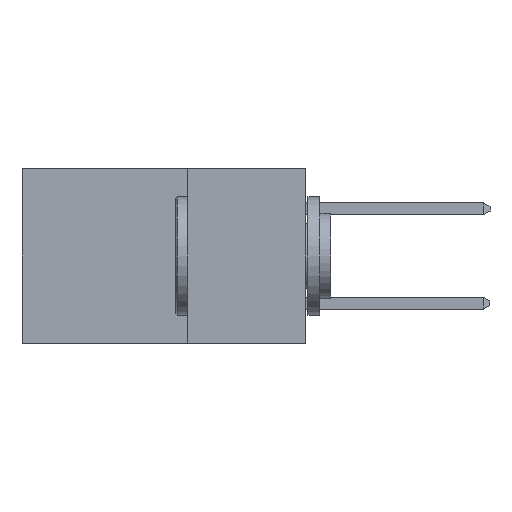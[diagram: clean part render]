
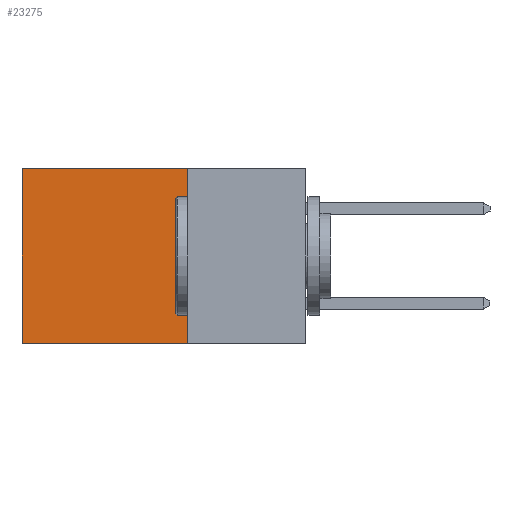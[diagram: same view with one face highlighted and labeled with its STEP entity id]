
A CAD part, left-side view. The second image highlights one B-rep face of the part: STEP entity #23275.
In plain terms, the highlighted planar face has unit normal (-1, 0, 0).
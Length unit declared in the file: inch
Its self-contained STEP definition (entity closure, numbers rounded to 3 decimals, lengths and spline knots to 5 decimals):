
#41 = ORIENTED_EDGE ( 'NONE', *, *, #3995, .F. ) ;
#1849 = CARTESIAN_POINT ( 'NONE',  ( 0.298, 0.25, 0. ) ) ;
#2735 = VERTEX_POINT ( 'NONE', #5864 ) ;
#3995 = EDGE_CURVE ( 'NONE', #4133, #2735, #20328, .T. ) ;
#4133 = VERTEX_POINT ( 'NONE', #1849 ) ;
#5017 = CARTESIAN_POINT ( 'NONE',  ( 0.298, 0.25, -0.37 ) ) ;
#5154 = ORIENTED_EDGE ( 'NONE', *, *, #13504, .T. ) ;
#5864 = CARTESIAN_POINT ( 'NONE',  ( 0.298, 0.25, -0.37 ) ) ;
#6428 = DIRECTION ( 'NONE',  ( 0., 1., 0. ) ) ;
#7084 = VECTOR ( 'NONE', #25562, 39.37008 ) ;
#7265 = DIRECTION ( 'NONE',  ( 0., 1., 0. ) ) ;
#7666 = VERTEX_POINT ( 'NONE', #19986 ) ;
#8743 = VECTOR ( 'NONE', #25901, 39.37008 ) ;
#9275 = ORIENTED_EDGE ( 'NONE', *, *, #20867, .F. ) ;
#10315 = VECTOR ( 'NONE', #6428, 39.37008 ) ;
#11048 = DIRECTION ( 'NONE',  ( 0., 0., -1. ) ) ;
#13504 = EDGE_CURVE ( 'NONE', #4133, #24951, #21853, .T. ) ;
#14989 = PLANE ( 'NONE',  #20465 ) ;
#16361 = CARTESIAN_POINT ( 'NONE',  ( 0.298, 0.6, 0. ) ) ;
#16399 = VECTOR ( 'NONE', #7265, 39.37008 ) ;
#16964 = CARTESIAN_POINT ( 'NONE',  ( 0.298, 0.6, 0. ) ) ;
#17722 = LINE ( 'NONE', #5017, #16399 ) ;
#18702 = LINE ( 'NONE', #16964, #7084 ) ;
#19986 = CARTESIAN_POINT ( 'NONE',  ( 0.298, 0.6, -0.37 ) ) ;
#20148 = EDGE_LOOP ( 'NONE', ( #22539, #9275, #41, #5154 ) ) ;
#20328 = LINE ( 'NONE', #27157, #8743 ) ;
#20465 = AXIS2_PLACEMENT_3D ( 'NONE', #21863, #23988, #11048 ) ;
#20867 = EDGE_CURVE ( 'NONE', #2735, #7666, #17722, .T. ) ;
#21656 = CARTESIAN_POINT ( 'NONE',  ( 0.298, 0.25, 0. ) ) ;
#21853 = LINE ( 'NONE', #21656, #10315 ) ;
#21859 = EDGE_CURVE ( 'NONE', #24951, #7666, #18702, .T. ) ;
#21863 = CARTESIAN_POINT ( 'NONE',  ( 0.298, 0.25, 0. ) ) ;
#22539 = ORIENTED_EDGE ( 'NONE', *, *, #21859, .T. ) ;
#23275 = ADVANCED_FACE ( 'NONE', ( #26599 ), #14989, .F. ) ;
#23988 = DIRECTION ( 'NONE',  ( 1., 0., 0. ) ) ;
#24951 = VERTEX_POINT ( 'NONE', #16361 ) ;
#25562 = DIRECTION ( 'NONE',  ( 0., 0., -1. ) ) ;
#25901 = DIRECTION ( 'NONE',  ( 0., 0., -1. ) ) ;
#26599 = FACE_OUTER_BOUND ( 'NONE', #20148, .T. ) ;
#27157 = CARTESIAN_POINT ( 'NONE',  ( 0.298, 0.25, 0. ) ) ;
